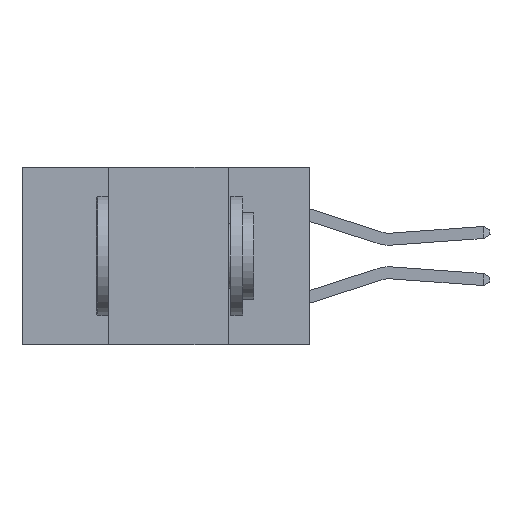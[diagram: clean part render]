
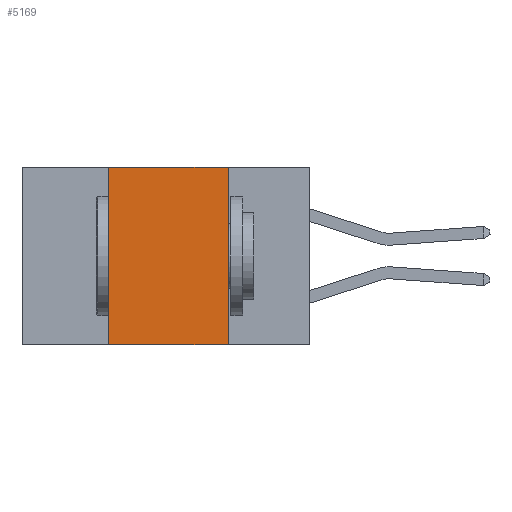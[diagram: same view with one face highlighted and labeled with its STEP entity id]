
A CAD part, left-side view. The second image highlights one B-rep face of the part: STEP entity #5169.
In plain terms, the highlighted planar face has unit normal (-1, 0, 0).
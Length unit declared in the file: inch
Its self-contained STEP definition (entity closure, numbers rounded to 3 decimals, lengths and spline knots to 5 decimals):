
#551 = EDGE_CURVE ( 'NONE', #3230, #7950, #15127, .T. ) ;
#708 = VECTOR ( 'NONE', #18510, 39.37008 ) ;
#823 = AXIS2_PLACEMENT_3D ( 'NONE', #18876, #18740, #3913 ) ;
#2182 = CARTESIAN_POINT ( 'NONE',  ( 0., 0.6, -0.37 ) ) ;
#2390 = VECTOR ( 'NONE', #16912, 39.37008 ) ;
#2499 = ORIENTED_EDGE ( 'NONE', *, *, #5252, .F. ) ;
#2565 = LINE ( 'NONE', #2182, #708 ) ;
#3230 = VERTEX_POINT ( 'NONE', #13370 ) ;
#3604 = LINE ( 'NONE', #17716, #9943 ) ;
#3913 = DIRECTION ( 'NONE',  ( 0., 0., -1. ) ) ;
#4081 = FACE_OUTER_BOUND ( 'NONE', #9322, .T. ) ;
#4090 = CARTESIAN_POINT ( 'NONE',  ( 0., 0.42, 0. ) ) ;
#4193 = VECTOR ( 'NONE', #13200, 39.37008 ) ;
#4920 = ORIENTED_EDGE ( 'NONE', *, *, #18859, .T. ) ;
#5169 = ADVANCED_FACE ( 'NONE', ( #4081 ), #18684, .F. ) ;
#5252 = EDGE_CURVE ( 'NONE', #7950, #12137, #3604, .T. ) ;
#7234 = VERTEX_POINT ( 'NONE', #12167 ) ;
#7950 = VERTEX_POINT ( 'NONE', #12540 ) ;
#8880 = ORIENTED_EDGE ( 'NONE', *, *, #17100, .F. ) ;
#9322 = EDGE_LOOP ( 'NONE', ( #2499, #17196, #8880, #4920 ) ) ;
#9943 = VECTOR ( 'NONE', #17523, 39.37008 ) ;
#10124 = CARTESIAN_POINT ( 'NONE',  ( 0., 0.6, 0. ) ) ;
#12137 = VERTEX_POINT ( 'NONE', #15254 ) ;
#12167 = CARTESIAN_POINT ( 'NONE',  ( 0., 0.42, -0.37 ) ) ;
#12212 = LINE ( 'NONE', #4090, #2390 ) ;
#12540 = CARTESIAN_POINT ( 'NONE',  ( 0., 0.17, 0. ) ) ;
#13200 = DIRECTION ( 'NONE',  ( 0., -1., 0. ) ) ;
#13370 = CARTESIAN_POINT ( 'NONE',  ( 0., 0.42, 0. ) ) ;
#15127 = LINE ( 'NONE', #10124, #4193 ) ;
#15254 = CARTESIAN_POINT ( 'NONE',  ( 0., 0.17, -0.37 ) ) ;
#16912 = DIRECTION ( 'NONE',  ( 0., 0., 1. ) ) ;
#17100 = EDGE_CURVE ( 'NONE', #7234, #3230, #12212, .T. ) ;
#17196 = ORIENTED_EDGE ( 'NONE', *, *, #551, .F. ) ;
#17523 = DIRECTION ( 'NONE',  ( 0., 0., -1. ) ) ;
#17716 = CARTESIAN_POINT ( 'NONE',  ( 0., 0.17, 0. ) ) ;
#18510 = DIRECTION ( 'NONE',  ( 0., -1., 0. ) ) ;
#18684 = PLANE ( 'NONE',  #823 ) ;
#18740 = DIRECTION ( 'NONE',  ( 1., 0., 0. ) ) ;
#18859 = EDGE_CURVE ( 'NONE', #7234, #12137, #2565, .T. ) ;
#18876 = CARTESIAN_POINT ( 'NONE',  ( 0., 0.6, 0. ) ) ;
